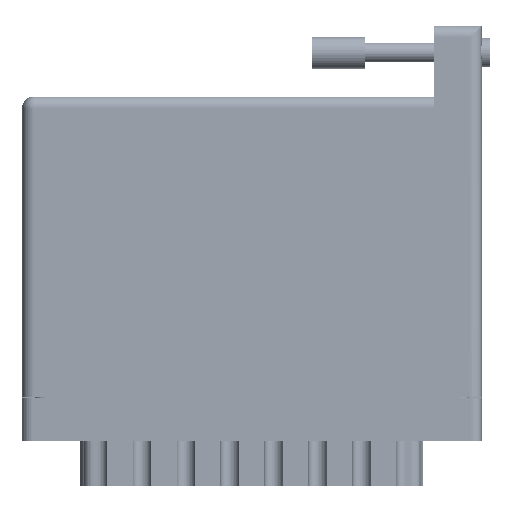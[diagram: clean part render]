
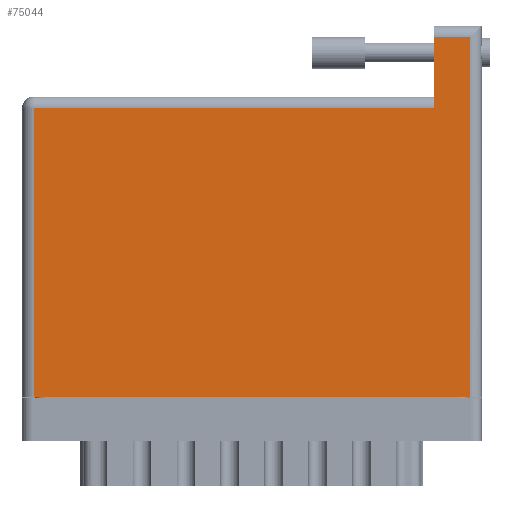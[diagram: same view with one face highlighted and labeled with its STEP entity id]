
A CAD part, front view. The second image highlights one B-rep face of the part: STEP entity #75044.
In plain terms, the highlighted face is planar.
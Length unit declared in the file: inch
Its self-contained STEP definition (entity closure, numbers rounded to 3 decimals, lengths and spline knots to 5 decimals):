
#1061 = CARTESIAN_POINT ( 'NONE',  ( 2.648, 0., 0. ) ) ;
#1901 = EDGE_CURVE ( 'NONE', #43257, #45625, #57669, .T. ) ;
#2152 = VECTOR ( 'NONE', #24340, 39.37008 ) ;
#3019 = VECTOR ( 'NONE', #54197, 39.37008 ) ;
#5649 = ORIENTED_EDGE ( 'NONE', *, *, #73450, .T. ) ;
#8802 = VECTOR ( 'NONE', #13055, 39.37008 ) ;
#11653 = DIRECTION ( 'NONE',  ( 0., 0., -1. ) ) ;
#12327 = DIRECTION ( 'NONE',  ( -1., 0., 0. ) ) ;
#13055 = DIRECTION ( 'NONE',  ( 0., 1., 0. ) ) ;
#18688 = LINE ( 'NONE', #55222, #3019 ) ;
#23922 = CARTESIAN_POINT ( 'NONE',  ( 0., 1.705, 0. ) ) ;
#24340 = DIRECTION ( 'NONE',  ( 0., -1., 0. ) ) ;
#25507 = VERTEX_POINT ( 'NONE', #48695 ) ;
#27949 = ORIENTED_EDGE ( 'NONE', *, *, #70612, .T. ) ;
#28572 = CARTESIAN_POINT ( 'NONE',  ( 2.438, 1.705, 0. ) ) ;
#28674 = AXIS2_PLACEMENT_3D ( 'NONE', #64149, #11653, #53083 ) ;
#29311 = LINE ( 'NONE', #50372, #69753 ) ;
#31460 = VERTEX_POINT ( 'NONE', #47472 ) ;
#35216 = EDGE_LOOP ( 'NONE', ( #5649, #41902, #61665, #56379, #66251, #27949 ) ) ;
#41902 = ORIENTED_EDGE ( 'NONE', *, *, #72125, .T. ) ;
#43257 = VERTEX_POINT ( 'NONE', #1061 ) ;
#44770 = VERTEX_POINT ( 'NONE', #71574 ) ;
#45287 = CARTESIAN_POINT ( 'NONE',  ( 2.648, 2.125, 0. ) ) ;
#45625 = VERTEX_POINT ( 'NONE', #45287 ) ;
#47260 = LINE ( 'NONE', #53694, #2152 ) ;
#47311 = EDGE_CURVE ( 'NONE', #31460, #43257, #29311, .T. ) ;
#47472 = CARTESIAN_POINT ( 'NONE',  ( 0.07, 0., 0. ) ) ;
#48695 = CARTESIAN_POINT ( 'NONE',  ( 0.07, 1.705, 0. ) ) ;
#50372 = CARTESIAN_POINT ( 'NONE',  ( 0., 0., 0. ) ) ;
#51576 = CARTESIAN_POINT ( 'NONE',  ( 2.438, 2.195, 0. ) ) ;
#53083 = DIRECTION ( 'NONE',  ( -1., 0., 0. ) ) ;
#53694 = CARTESIAN_POINT ( 'NONE',  ( 0.07, 0., 0. ) ) ;
#54197 = DIRECTION ( 'NONE',  ( -1., 0., 0. ) ) ;
#55222 = CARTESIAN_POINT ( 'NONE',  ( 0., 2.125, 0. ) ) ;
#56379 = ORIENTED_EDGE ( 'NONE', *, *, #1901, .T. ) ;
#57669 = LINE ( 'NONE', #63012, #8802 ) ;
#58634 = LINE ( 'NONE', #51576, #74224 ) ;
#60163 = FACE_OUTER_BOUND ( 'NONE', #35216, .T. ) ;
#61665 = ORIENTED_EDGE ( 'NONE', *, *, #47311, .T. ) ;
#63012 = CARTESIAN_POINT ( 'NONE',  ( 2.648, 2.195, 0. ) ) ;
#63393 = DIRECTION ( 'NONE',  ( 0., -1., 0. ) ) ;
#64149 = CARTESIAN_POINT ( 'NONE',  ( 0., 1.775, 0. ) ) ;
#64795 = VECTOR ( 'NONE', #12327, 39.37008 ) ;
#66251 = ORIENTED_EDGE ( 'NONE', *, *, #74149, .T. ) ;
#67837 = DIRECTION ( 'NONE',  ( 1., 0., 0. ) ) ;
#68192 = VERTEX_POINT ( 'NONE', #28572 ) ;
#69753 = VECTOR ( 'NONE', #67837, 39.37008 ) ;
#70612 = EDGE_CURVE ( 'NONE', #44770, #68192, #58634, .T. ) ;
#71574 = CARTESIAN_POINT ( 'NONE',  ( 2.438, 2.125, 0. ) ) ;
#72125 = EDGE_CURVE ( 'NONE', #25507, #31460, #47260, .T. ) ;
#73450 = EDGE_CURVE ( 'NONE', #68192, #25507, #75876, .T. ) ;
#74149 = EDGE_CURVE ( 'NONE', #45625, #44770, #18688, .T. ) ;
#74224 = VECTOR ( 'NONE', #63393, 39.37008 ) ;
#75044 = ADVANCED_FACE ( 'NONE', ( #60163 ), #75711, .F. ) ;
#75711 = PLANE ( 'NONE',  #28674 ) ;
#75876 = LINE ( 'NONE', #23922, #64795 ) ;
